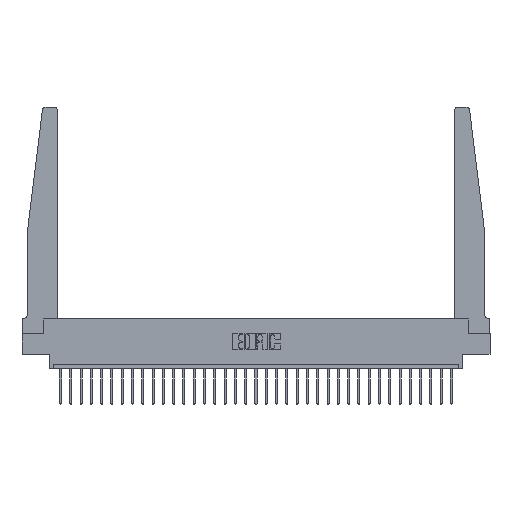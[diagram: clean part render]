
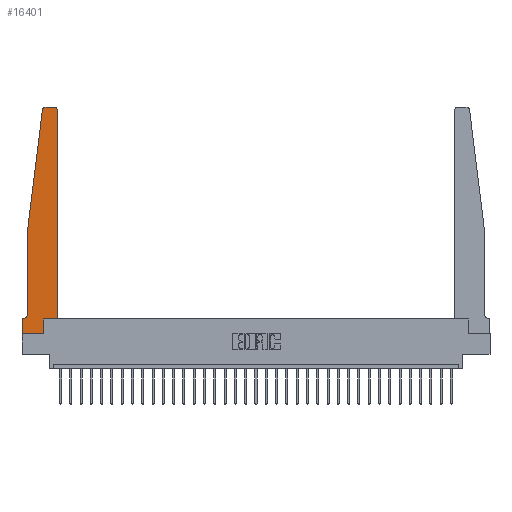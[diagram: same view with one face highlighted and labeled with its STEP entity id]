
A CAD part, top view. The second image highlights one B-rep face of the part: STEP entity #16401.
In plain terms, the highlighted planar face has unit normal (0, 0, 1).
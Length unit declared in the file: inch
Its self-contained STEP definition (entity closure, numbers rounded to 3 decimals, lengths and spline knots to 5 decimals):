
#250 = DIRECTION ( 'NONE',  ( 0., 0., 1. ) ) ;
#712 = EDGE_CURVE ( 'NONE', #15908, #23615, #1759, .T. ) ;
#1157 = DIRECTION ( 'NONE',  ( -1., 0., 0. ) ) ;
#1158 = EDGE_CURVE ( 'NONE', #11933, #20254, #2440, .T. ) ;
#1282 = EDGE_CURVE ( 'NONE', #17860, #5711, #6364, .T. ) ;
#1348 = CARTESIAN_POINT ( 'NONE',  ( 0.065, 0.1875, 0.37 ) ) ;
#1572 = ORIENTED_EDGE ( 'NONE', *, *, #20629, .T. ) ;
#1759 = CIRCLE ( 'NONE', #6559, 0.05 ) ;
#2440 = LINE ( 'NONE', #16933, #25974 ) ;
#2755 = DIRECTION ( 'NONE',  ( -1., 0., 0. ) ) ;
#2763 = EDGE_CURVE ( 'NONE', #15959, #17521, #8471, .T. ) ;
#3061 = CARTESIAN_POINT ( 'NONE',  ( 0.015, 0.2375, 0.37 ) ) ;
#3825 = EDGE_CURVE ( 'NONE', #5711, #15098, #21232, .T. ) ;
#4028 = DIRECTION ( 'NONE',  ( 1., 0., 0. ) ) ;
#4043 = EDGE_CURVE ( 'NONE', #15098, #27141, #24036, .T. ) ;
#4572 = CARTESIAN_POINT ( 'NONE',  ( 0., 0.1875, 0.37 ) ) ;
#5141 = CARTESIAN_POINT ( 'NONE',  ( 0.395, 2.72, 0.37 ) ) ;
#5337 = DIRECTION ( 'NONE',  ( 0., 0., -1. ) ) ;
#5711 = VERTEX_POINT ( 'NONE', #17412 ) ;
#5863 = VECTOR ( 'NONE', #17811, 39.37008 ) ;
#6231 = ORIENTED_EDGE ( 'NONE', *, *, #21194, .T. ) ;
#6364 = LINE ( 'NONE', #15391, #8505 ) ;
#6559 = AXIS2_PLACEMENT_3D ( 'NONE', #3061, #5337, #2755 ) ;
#6706 = CARTESIAN_POINT ( 'NONE',  ( 0.27653, 2.75, 0.37 ) ) ;
#6739 = AXIS2_PLACEMENT_3D ( 'NONE', #4572, #13906, #20427 ) ;
#7152 = ORIENTED_EDGE ( 'NONE', *, *, #3825, .T. ) ;
#7563 = VECTOR ( 'NONE', #1157, 39.37008 ) ;
#8471 = LINE ( 'NONE', #9717, #19882 ) ;
#8505 = VECTOR ( 'NONE', #4028, 39.37008 ) ;
#8876 = FACE_OUTER_BOUND ( 'NONE', #10177, .T. ) ;
#9063 = DIRECTION ( 'NONE',  ( 0., 1., 0. ) ) ;
#9090 = VECTOR ( 'NONE', #14628, 39.37008 ) ;
#9163 = CIRCLE ( 'NONE', #19727, 0.03 ) ;
#9717 = CARTESIAN_POINT ( 'NONE',  ( 0.065, 1.25, 0.37 ) ) ;
#10052 = EDGE_CURVE ( 'NONE', #17521, #15908, #19854, .T. ) ;
#10113 = DIRECTION ( 'NONE',  ( -0.122, -0.992, 0. ) ) ;
#10177 = EDGE_LOOP ( 'NONE', ( #18313, #26136, #24714, #12645, #17644, #1572, #22864, #15804, #7152, #21664, #6231, #18694 ) ) ;
#10694 = CARTESIAN_POINT ( 'NONE',  ( 0.425, 0.18, 0.37 ) ) ;
#11933 = VERTEX_POINT ( 'NONE', #19995 ) ;
#12106 = CARTESIAN_POINT ( 'NONE',  ( 0.2605, 0.18, 0.37 ) ) ;
#12645 = ORIENTED_EDGE ( 'NONE', *, *, #10052, .T. ) ;
#13226 = CARTESIAN_POINT ( 'NONE',  ( 0.27653, 2.72, 0.37 ) ) ;
#13906 = DIRECTION ( 'NONE',  ( 0., 0., 1. ) ) ;
#14300 = DIRECTION ( 'NONE',  ( 0., -1., 0. ) ) ;
#14628 = DIRECTION ( 'NONE',  ( 0., 1., 0. ) ) ;
#15098 = VERTEX_POINT ( 'NONE', #25519 ) ;
#15279 = CARTESIAN_POINT ( 'NONE',  ( 0.425, 2.72, 0.37 ) ) ;
#15391 = CARTESIAN_POINT ( 'NONE',  ( 0., 0., 0.37 ) ) ;
#15615 = CARTESIAN_POINT ( 'NONE',  ( 0.425, 0.18, 0.37 ) ) ;
#15692 = EDGE_CURVE ( 'NONE', #20254, #15959, #29236, .T. ) ;
#15804 = ORIENTED_EDGE ( 'NONE', *, *, #1282, .T. ) ;
#15908 = VERTEX_POINT ( 'NONE', #28260 ) ;
#15959 = VERTEX_POINT ( 'NONE', #28453 ) ;
#16117 = CARTESIAN_POINT ( 'NONE',  ( 0., 0., 0.37 ) ) ;
#16401 = ADVANCED_FACE ( 'NONE', ( #8876 ), #18220, .T. ) ;
#16776 = VERTEX_POINT ( 'NONE', #26260 ) ;
#16933 = CARTESIAN_POINT ( 'NONE',  ( 0.25, 2.75, 0.37 ) ) ;
#16998 = EDGE_CURVE ( 'NONE', #16776, #17860, #20967, .T. ) ;
#17412 = CARTESIAN_POINT ( 'NONE',  ( 0.2605, 0., 0.37 ) ) ;
#17433 = DIRECTION ( 'NONE',  ( 0., 0., 1. ) ) ;
#17521 = VERTEX_POINT ( 'NONE', #28257 ) ;
#17644 = ORIENTED_EDGE ( 'NONE', *, *, #712, .T. ) ;
#17811 = DIRECTION ( 'NONE',  ( 1., 0., 0. ) ) ;
#17860 = VERTEX_POINT ( 'NONE', #25964 ) ;
#18220 = PLANE ( 'NONE',  #6739 ) ;
#18313 = ORIENTED_EDGE ( 'NONE', *, *, #1158, .T. ) ;
#18694 = ORIENTED_EDGE ( 'NONE', *, *, #26359, .T. ) ;
#19727 = AXIS2_PLACEMENT_3D ( 'NONE', #5141, #250, #25270 ) ;
#19854 = LINE ( 'NONE', #26176, #22707 ) ;
#19882 = VECTOR ( 'NONE', #10113, 39.37008 ) ;
#19995 = CARTESIAN_POINT ( 'NONE',  ( 0.395, 2.75, 0.37 ) ) ;
#20254 = VERTEX_POINT ( 'NONE', #6706 ) ;
#20408 = VECTOR ( 'NONE', #9063, 39.37008 ) ;
#20427 = DIRECTION ( 'NONE',  ( 1., 0., 0. ) ) ;
#20539 = CARTESIAN_POINT ( 'NONE',  ( 0.425, 0.18, 0.37 ) ) ;
#20627 = VECTOR ( 'NONE', #14300, 39.37008 ) ;
#20629 = EDGE_CURVE ( 'NONE', #23615, #16776, #27894, .T. ) ;
#20967 = LINE ( 'NONE', #16117, #20627 ) ;
#21194 = EDGE_CURVE ( 'NONE', #27141, #24060, #26445, .T. ) ;
#21232 = LINE ( 'NONE', #12106, #9090 ) ;
#21664 = ORIENTED_EDGE ( 'NONE', *, *, #4043, .T. ) ;
#22707 = VECTOR ( 'NONE', #28473, 39.37008 ) ;
#22864 = ORIENTED_EDGE ( 'NONE', *, *, #16998, .T. ) ;
#23615 = VERTEX_POINT ( 'NONE', #23695 ) ;
#23695 = CARTESIAN_POINT ( 'NONE',  ( 0.015, 0.1875, 0.37 ) ) ;
#24036 = LINE ( 'NONE', #15615, #5863 ) ;
#24060 = VERTEX_POINT ( 'NONE', #15279 ) ;
#24714 = ORIENTED_EDGE ( 'NONE', *, *, #2763, .T. ) ;
#25270 = DIRECTION ( 'NONE',  ( 1., 0., 0. ) ) ;
#25519 = CARTESIAN_POINT ( 'NONE',  ( 0.2605, 0.18, 0.37 ) ) ;
#25964 = CARTESIAN_POINT ( 'NONE',  ( 0., 0., 0.37 ) ) ;
#25974 = VECTOR ( 'NONE', #28582, 39.37008 ) ;
#26136 = ORIENTED_EDGE ( 'NONE', *, *, #15692, .T. ) ;
#26176 = CARTESIAN_POINT ( 'NONE',  ( 0.065, 1.25, 0.37 ) ) ;
#26260 = CARTESIAN_POINT ( 'NONE',  ( 0., 0.1875, 0.37 ) ) ;
#26359 = EDGE_CURVE ( 'NONE', #24060, #11933, #9163, .T. ) ;
#26445 = LINE ( 'NONE', #20539, #20408 ) ;
#27141 = VERTEX_POINT ( 'NONE', #10694 ) ;
#27894 = LINE ( 'NONE', #1348, #7563 ) ;
#28257 = CARTESIAN_POINT ( 'NONE',  ( 0.065, 1.25, 0.37 ) ) ;
#28260 = CARTESIAN_POINT ( 'NONE',  ( 0.065, 0.2375, 0.37 ) ) ;
#28453 = CARTESIAN_POINT ( 'NONE',  ( 0.24675, 2.72367, 0.37 ) ) ;
#28471 = AXIS2_PLACEMENT_3D ( 'NONE', #13226, #17433, #29178 ) ;
#28473 = DIRECTION ( 'NONE',  ( 0., -1., 0. ) ) ;
#28582 = DIRECTION ( 'NONE',  ( -1., 0., 0. ) ) ;
#29178 = DIRECTION ( 'NONE',  ( 1., 0., 0. ) ) ;
#29236 = CIRCLE ( 'NONE', #28471, 0.03 ) ;
